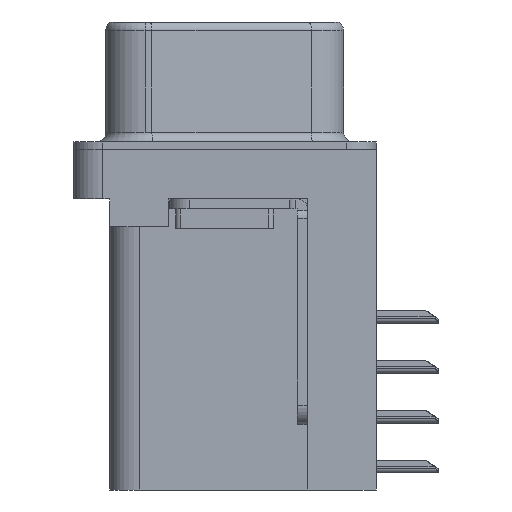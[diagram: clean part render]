
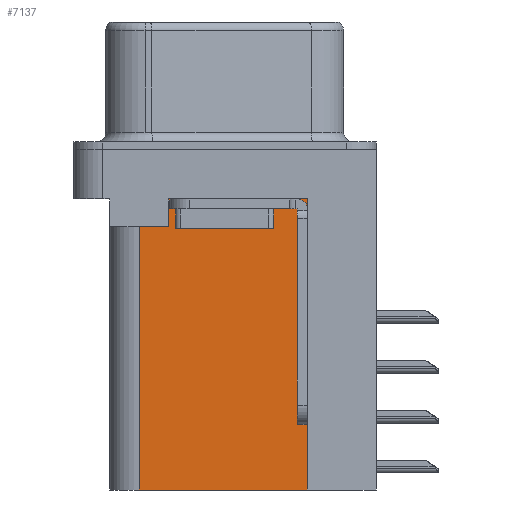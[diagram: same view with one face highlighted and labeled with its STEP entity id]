
A CAD part, left-side view. The second image highlights one B-rep face of the part: STEP entity #7137.
In plain terms, the highlighted planar face has unit normal (-1, 0, 0).
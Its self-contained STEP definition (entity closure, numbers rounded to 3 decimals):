
#143 = DIRECTION ( 'NONE',  ( 0., 0., -1. ) ) ;
#515 = AXIS2_PLACEMENT_3D ( 'NONE', #12427, #34768, #15611 ) ;
#553 = VECTOR ( 'NONE', #39598, 1000. ) ;
#997 = VECTOR ( 'NONE', #34887, 1000. ) ;
#2516 = ORIENTED_EDGE ( 'NONE', *, *, #23051, .T. ) ;
#3660 = LINE ( 'NONE', #26217, #19624 ) ;
#4487 = VECTOR ( 'NONE', #23868, 1000. ) ;
#6275 = EDGE_LOOP ( 'NONE', ( #15740, #24534, #2516, #8535, #20845, #14697 ) ) ;
#6542 = VERTEX_POINT ( 'NONE', #39065 ) ;
#7137 = ADVANCED_FACE ( 'NONE', ( #39820 ), #25112, .F. ) ;
#8001 = CARTESIAN_POINT ( 'NONE',  ( 3.75, -4.2, -2.5 ) ) ;
#8165 = VERTEX_POINT ( 'NONE', #37569 ) ;
#8535 = ORIENTED_EDGE ( 'NONE', *, *, #32292, .F. ) ;
#8928 = CARTESIAN_POINT ( 'NONE',  ( 3.75, 4.35, -3.9 ) ) ;
#9061 = LINE ( 'NONE', #14024, #553 ) ;
#12427 = CARTESIAN_POINT ( 'NONE',  ( 3.75, -4.2, -17.3 ) ) ;
#12469 = VECTOR ( 'NONE', #143, 1000. ) ;
#12554 = CARTESIAN_POINT ( 'NONE',  ( 3.75, -4.2, -17.3 ) ) ;
#13288 = EDGE_CURVE ( 'NONE', #8165, #15123, #37945, .T. ) ;
#13708 = DIRECTION ( 'NONE',  ( 0., 1., 0. ) ) ;
#14024 = CARTESIAN_POINT ( 'NONE',  ( 3.75, 4.35, -17.3 ) ) ;
#14697 = ORIENTED_EDGE ( 'NONE', *, *, #34030, .T. ) ;
#15123 = VERTEX_POINT ( 'NONE', #22700 ) ;
#15611 = DIRECTION ( 'NONE',  ( 0., 1., 0. ) ) ;
#15740 = ORIENTED_EDGE ( 'NONE', *, *, #35947, .T. ) ;
#19624 = VECTOR ( 'NONE', #29432, 1000. ) ;
#20124 = CARTESIAN_POINT ( 'NONE',  ( 3.75, 0., -3.9 ) ) ;
#20845 = ORIENTED_EDGE ( 'NONE', *, *, #36584, .F. ) ;
#21415 = LINE ( 'NONE', #8001, #4487 ) ;
#22700 = CARTESIAN_POINT ( 'NONE',  ( 3.75, 2.85, -3.9 ) ) ;
#23051 = EDGE_CURVE ( 'NONE', #15123, #33842, #28775, .T. ) ;
#23868 = DIRECTION ( 'NONE',  ( 0., 1., 0. ) ) ;
#24445 = LINE ( 'NONE', #12554, #997 ) ;
#24534 = ORIENTED_EDGE ( 'NONE', *, *, #13288, .T. ) ;
#25112 = PLANE ( 'NONE',  #515 ) ;
#26217 = CARTESIAN_POINT ( 'NONE',  ( 3.75, -4.2, -17.3 ) ) ;
#26481 = VERTEX_POINT ( 'NONE', #35477 ) ;
#28775 = LINE ( 'NONE', #20124, #29780 ) ;
#29432 = DIRECTION ( 'NONE',  ( 0., 0., 1. ) ) ;
#29780 = VECTOR ( 'NONE', #13708, 1000. ) ;
#32292 = EDGE_CURVE ( 'NONE', #26481, #33842, #9061, .T. ) ;
#33842 = VERTEX_POINT ( 'NONE', #8928 ) ;
#34030 = EDGE_CURVE ( 'NONE', #6542, #36856, #3660, .T. ) ;
#34768 = DIRECTION ( 'NONE',  ( 1., 0., 0. ) ) ;
#34887 = DIRECTION ( 'NONE',  ( 0., 1., 0. ) ) ;
#35477 = CARTESIAN_POINT ( 'NONE',  ( 3.75, 4.35, -17.3 ) ) ;
#35947 = EDGE_CURVE ( 'NONE', #36856, #8165, #21415, .T. ) ;
#36584 = EDGE_CURVE ( 'NONE', #6542, #26481, #24445, .T. ) ;
#36856 = VERTEX_POINT ( 'NONE', #39194 ) ;
#37569 = CARTESIAN_POINT ( 'NONE',  ( 3.75, 2.85, -2.5 ) ) ;
#37945 = LINE ( 'NONE', #38369, #12469 ) ;
#38369 = CARTESIAN_POINT ( 'NONE',  ( 3.75, 2.85, -3.9 ) ) ;
#39065 = CARTESIAN_POINT ( 'NONE',  ( 3.75, -4.2, -17.3 ) ) ;
#39194 = CARTESIAN_POINT ( 'NONE',  ( 3.75, -4.2, -2.5 ) ) ;
#39598 = DIRECTION ( 'NONE',  ( 0., 0., 1. ) ) ;
#39820 = FACE_OUTER_BOUND ( 'NONE', #6275, .T. ) ;
